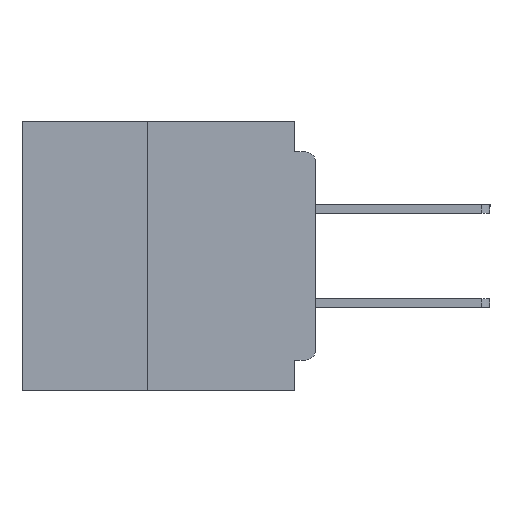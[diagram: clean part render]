
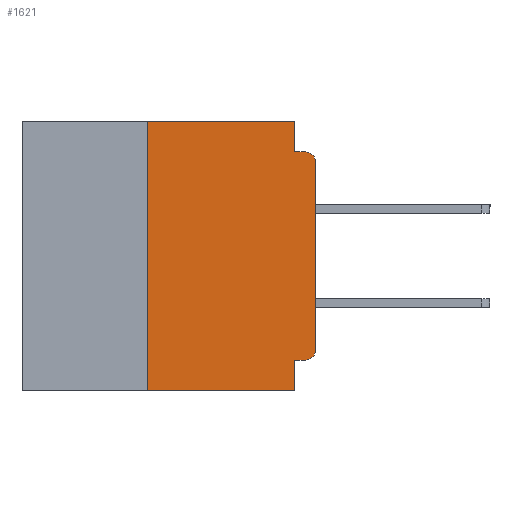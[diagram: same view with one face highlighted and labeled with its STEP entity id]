
A CAD part, left-side view. The second image highlights one B-rep face of the part: STEP entity #1621.
In plain terms, the highlighted planar face has unit normal (-1, 0, 0).
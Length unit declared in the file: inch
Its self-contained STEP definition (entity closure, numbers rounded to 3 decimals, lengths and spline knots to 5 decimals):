
#898 = VECTOR ( 'NONE', #24856, 39.37008 ) ;
#1201 = VECTOR ( 'NONE', #13776, 39.37008 ) ;
#1317 = VERTEX_POINT ( 'NONE', #49202 ) ;
#1621 = ADVANCED_FACE ( 'NONE', ( #12761 ), #17134, .F. ) ;
#1766 = CARTESIAN_POINT ( 'NONE',  ( 0., 0.015, -0.06 ) ) ;
#1852 = VECTOR ( 'NONE', #11097, 39.37008 ) ;
#5743 = VECTOR ( 'NONE', #31219, 39.37008 ) ;
#6525 = LINE ( 'NONE', #60457, #1852 ) ;
#6763 = DIRECTION ( 'NONE',  ( 0., 0., -1. ) ) ;
#7667 = LINE ( 'NONE', #9147, #48768 ) ;
#9106 = DIRECTION ( 'NONE',  ( -1., 0., 0. ) ) ;
#9147 = CARTESIAN_POINT ( 'NONE',  ( 0., 0., -0.045 ) ) ;
#9418 = EDGE_CURVE ( 'NONE', #21393, #49713, #49944, .T. ) ;
#9677 = VERTEX_POINT ( 'NONE', #43147 ) ;
#9850 = CARTESIAN_POINT ( 'NONE',  ( 0., 0.015, -0.045 ) ) ;
#10027 = CARTESIAN_POINT ( 'NONE',  ( 0., 0.031, -0.4 ) ) ;
#10318 = ORIENTED_EDGE ( 'NONE', *, *, #20987, .F. ) ;
#10664 = CARTESIAN_POINT ( 'NONE',  ( 0., 0.015, -0.355 ) ) ;
#11097 = DIRECTION ( 'NONE',  ( 0., 0., 1. ) ) ;
#12458 = VERTEX_POINT ( 'NONE', #44684 ) ;
#12761 = FACE_OUTER_BOUND ( 'NONE', #45715, .T. ) ;
#13328 = CIRCLE ( 'NONE', #24603, 0.015 ) ;
#13659 = EDGE_CURVE ( 'NONE', #59315, #61138, #53667, .T. ) ;
#13776 = DIRECTION ( 'NONE',  ( 0., 1., 0. ) ) ;
#14430 = LINE ( 'NONE', #23753, #1201 ) ;
#16695 = DIRECTION ( 'NONE',  ( 0., 0., -1. ) ) ;
#17121 = DIRECTION ( 'NONE',  ( 1., 0., 0. ) ) ;
#17134 = PLANE ( 'NONE',  #47609 ) ;
#17559 = CARTESIAN_POINT ( 'NONE',  ( 0., 0.437, 0. ) ) ;
#19553 = VERTEX_POINT ( 'NONE', #9850 ) ;
#19951 = AXIS2_PLACEMENT_3D ( 'NONE', #1766, #36425, #6763 ) ;
#20987 = EDGE_CURVE ( 'NONE', #59315, #12458, #6525, .T. ) ;
#21393 = VERTEX_POINT ( 'NONE', #48985 ) ;
#22263 = DIRECTION ( 'NONE',  ( 0., 0., 1. ) ) ;
#23707 = EDGE_CURVE ( 'NONE', #49713, #19553, #7667, .T. ) ;
#23753 = CARTESIAN_POINT ( 'NONE',  ( 0., 0., -0.355 ) ) ;
#24603 = AXIS2_PLACEMENT_3D ( 'NONE', #38820, #9106, #43786 ) ;
#24856 = DIRECTION ( 'NONE',  ( 0., -1., 0. ) ) ;
#25082 = ORIENTED_EDGE ( 'NONE', *, *, #13659, .T. ) ;
#26289 = CARTESIAN_POINT ( 'NONE',  ( 0., 0.031, 0. ) ) ;
#28189 = ORIENTED_EDGE ( 'NONE', *, *, #60644, .F. ) ;
#29220 = EDGE_CURVE ( 'NONE', #47098, #9677, #13328, .T. ) ;
#29719 = ORIENTED_EDGE ( 'NONE', *, *, #62187, .F. ) ;
#31219 = DIRECTION ( 'NONE',  ( 0., 0., -1. ) ) ;
#31995 = ORIENTED_EDGE ( 'NONE', *, *, #57648, .T. ) ;
#32246 = LINE ( 'NONE', #57235, #57053 ) ;
#33820 = DIRECTION ( 'NONE',  ( 0., -1., 0. ) ) ;
#33932 = LINE ( 'NONE', #36937, #44044 ) ;
#34253 = CARTESIAN_POINT ( 'NONE',  ( 0., 0., -0.06 ) ) ;
#36425 = DIRECTION ( 'NONE',  ( -1., 0., 0. ) ) ;
#36937 = CARTESIAN_POINT ( 'NONE',  ( 0., 0., 0. ) ) ;
#37402 = ORIENTED_EDGE ( 'NONE', *, *, #23707, .F. ) ;
#38557 = CARTESIAN_POINT ( 'NONE',  ( 0., 0.25, -0.4 ) ) ;
#38820 = CARTESIAN_POINT ( 'NONE',  ( 0., 0.015, -0.34 ) ) ;
#39568 = CARTESIAN_POINT ( 'NONE',  ( 0., 0.437, -0.4 ) ) ;
#42088 = ORIENTED_EDGE ( 'NONE', *, *, #9418, .F. ) ;
#43147 = CARTESIAN_POINT ( 'NONE',  ( 0., 0., -0.34 ) ) ;
#43786 = DIRECTION ( 'NONE',  ( 0., 0., -1. ) ) ;
#44044 = VECTOR ( 'NONE', #22263, 39.37008 ) ;
#44684 = CARTESIAN_POINT ( 'NONE',  ( 0., 0.25, 0. ) ) ;
#45278 = ORIENTED_EDGE ( 'NONE', *, *, #29220, .T. ) ;
#45715 = EDGE_LOOP ( 'NONE', ( #31995, #49058, #37402, #42088, #56802, #10318, #25082, #28189, #29719, #45278 ) ) ;
#47098 = VERTEX_POINT ( 'NONE', #10664 ) ;
#47609 = AXIS2_PLACEMENT_3D ( 'NONE', #17559, #17121, #16695 ) ;
#48768 = VECTOR ( 'NONE', #33820, 39.37008 ) ;
#48985 = CARTESIAN_POINT ( 'NONE',  ( 0., 0.031, 0. ) ) ;
#49058 = ORIENTED_EDGE ( 'NONE', *, *, #56468, .T. ) ;
#49202 = CARTESIAN_POINT ( 'NONE',  ( 0., 0.031, -0.355 ) ) ;
#49462 = DIRECTION ( 'NONE',  ( 0., 0., -1. ) ) ;
#49713 = VERTEX_POINT ( 'NONE', #53698 ) ;
#49944 = LINE ( 'NONE', #26289, #5743 ) ;
#52309 = DIRECTION ( 'NONE',  ( 0., -1., 0. ) ) ;
#53667 = LINE ( 'NONE', #39568, #898 ) ;
#53698 = CARTESIAN_POINT ( 'NONE',  ( 0., 0.031, -0.045 ) ) ;
#56468 = EDGE_CURVE ( 'NONE', #58764, #19553, #63413, .T. ) ;
#56475 = VECTOR ( 'NONE', #49462, 39.37008 ) ;
#56802 = ORIENTED_EDGE ( 'NONE', *, *, #58538, .F. ) ;
#57053 = VECTOR ( 'NONE', #52309, 39.37008 ) ;
#57235 = CARTESIAN_POINT ( 'NONE',  ( 0., 0.437, 0. ) ) ;
#57648 = EDGE_CURVE ( 'NONE', #9677, #58764, #33932, .T. ) ;
#58004 = LINE ( 'NONE', #10027, #56475 ) ;
#58538 = EDGE_CURVE ( 'NONE', #12458, #21393, #32246, .T. ) ;
#58764 = VERTEX_POINT ( 'NONE', #34253 ) ;
#59315 = VERTEX_POINT ( 'NONE', #38557 ) ;
#59538 = CARTESIAN_POINT ( 'NONE',  ( 0., 0.031, -0.4 ) ) ;
#60457 = CARTESIAN_POINT ( 'NONE',  ( 0., 0.25, -0.4 ) ) ;
#60644 = EDGE_CURVE ( 'NONE', #1317, #61138, #58004, .T. ) ;
#61138 = VERTEX_POINT ( 'NONE', #59538 ) ;
#62187 = EDGE_CURVE ( 'NONE', #47098, #1317, #14430, .T. ) ;
#63413 = CIRCLE ( 'NONE', #19951, 0.015 ) ;
